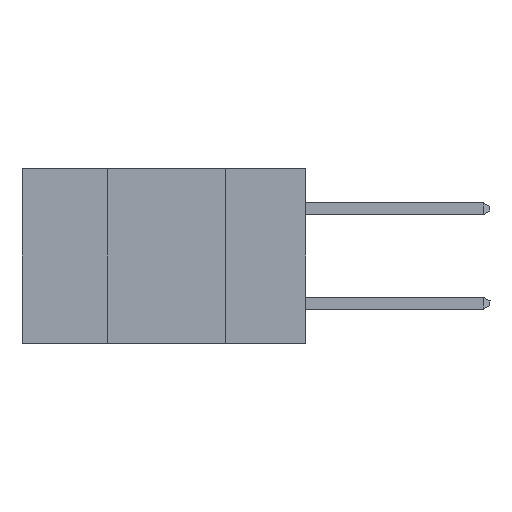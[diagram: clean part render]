
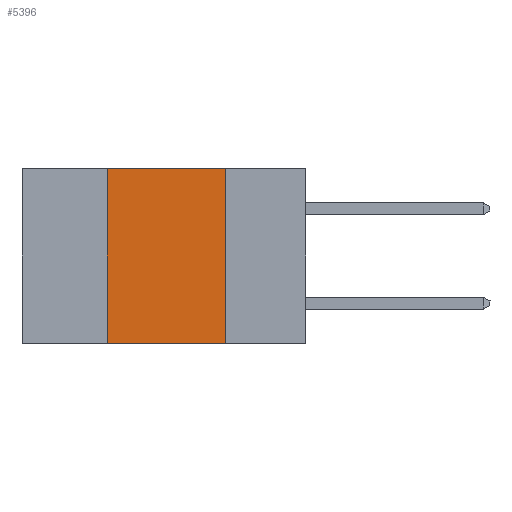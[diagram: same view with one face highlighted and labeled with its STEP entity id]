
A CAD part, left-side view. The second image highlights one B-rep face of the part: STEP entity #5396.
In plain terms, the highlighted planar face has unit normal (-1, 0, 0).
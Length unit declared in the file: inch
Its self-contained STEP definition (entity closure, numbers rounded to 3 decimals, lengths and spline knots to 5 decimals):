
#239 = EDGE_CURVE ( 'NONE', #1254, #1089, #5371, .T. ) ;
#408 = CARTESIAN_POINT ( 'NONE',  ( 0., 0.17, -0.37 ) ) ;
#464 = ORIENTED_EDGE ( 'NONE', *, *, #2790, .F. ) ;
#656 = DIRECTION ( 'NONE',  ( 0., 0., -1. ) ) ;
#1089 = VERTEX_POINT ( 'NONE', #8102 ) ;
#1254 = VERTEX_POINT ( 'NONE', #6616 ) ;
#1538 = ORIENTED_EDGE ( 'NONE', *, *, #239, .F. ) ;
#1543 = DIRECTION ( 'NONE',  ( 0., -1., 0. ) ) ;
#1554 = CARTESIAN_POINT ( 'NONE',  ( 0., 0.42, -0.37 ) ) ;
#2522 = DIRECTION ( 'NONE',  ( 0., 0., 1. ) ) ;
#2790 = EDGE_CURVE ( 'NONE', #5488, #1254, #9579, .T. ) ;
#2893 = DIRECTION ( 'NONE',  ( 0., -1., 0. ) ) ;
#3095 = PLANE ( 'NONE',  #7522 ) ;
#4051 = DIRECTION ( 'NONE',  ( 1., 0., 0. ) ) ;
#4071 = VECTOR ( 'NONE', #2522, 39.37008 ) ;
#4131 = ORIENTED_EDGE ( 'NONE', *, *, #9593, .F. ) ;
#4337 = ORIENTED_EDGE ( 'NONE', *, *, #4870, .T. ) ;
#4580 = LINE ( 'NONE', #10821, #5948 ) ;
#4643 = VECTOR ( 'NONE', #656, 39.37008 ) ;
#4870 = EDGE_CURVE ( 'NONE', #5488, #7322, #4580, .T. ) ;
#4952 = DIRECTION ( 'NONE',  ( 0., 0., -1. ) ) ;
#5163 = CARTESIAN_POINT ( 'NONE',  ( 0., 0.42, 0. ) ) ;
#5371 = LINE ( 'NONE', #7762, #9778 ) ;
#5396 = ADVANCED_FACE ( 'NONE', ( #9111 ), #3095, .F. ) ;
#5488 = VERTEX_POINT ( 'NONE', #1554 ) ;
#5948 = VECTOR ( 'NONE', #2893, 39.37008 ) ;
#6616 = CARTESIAN_POINT ( 'NONE',  ( 0., 0.42, 0. ) ) ;
#6688 = CARTESIAN_POINT ( 'NONE',  ( 0., 0.6, 0. ) ) ;
#7322 = VERTEX_POINT ( 'NONE', #408 ) ;
#7522 = AXIS2_PLACEMENT_3D ( 'NONE', #6688, #4051, #4952 ) ;
#7762 = CARTESIAN_POINT ( 'NONE',  ( 0., 0.6, 0. ) ) ;
#7833 = EDGE_LOOP ( 'NONE', ( #4131, #1538, #464, #4337 ) ) ;
#8102 = CARTESIAN_POINT ( 'NONE',  ( 0., 0.17, 0. ) ) ;
#9111 = FACE_OUTER_BOUND ( 'NONE', #7833, .T. ) ;
#9579 = LINE ( 'NONE', #5163, #4071 ) ;
#9593 = EDGE_CURVE ( 'NONE', #1089, #7322, #10158, .T. ) ;
#9691 = CARTESIAN_POINT ( 'NONE',  ( 0., 0.17, 0. ) ) ;
#9778 = VECTOR ( 'NONE', #1543, 39.37008 ) ;
#10158 = LINE ( 'NONE', #9691, #4643 ) ;
#10821 = CARTESIAN_POINT ( 'NONE',  ( 0., 0.6, -0.37 ) ) ;
